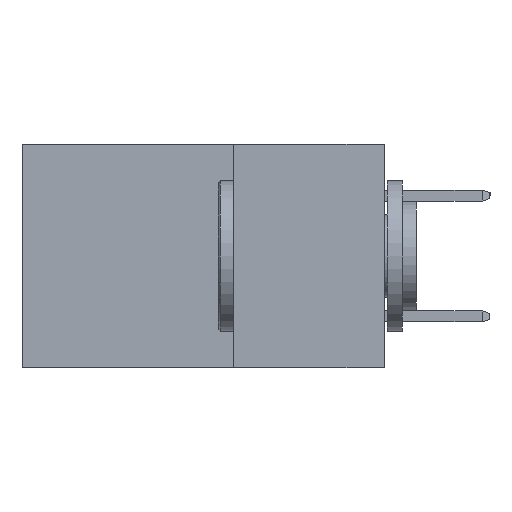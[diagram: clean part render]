
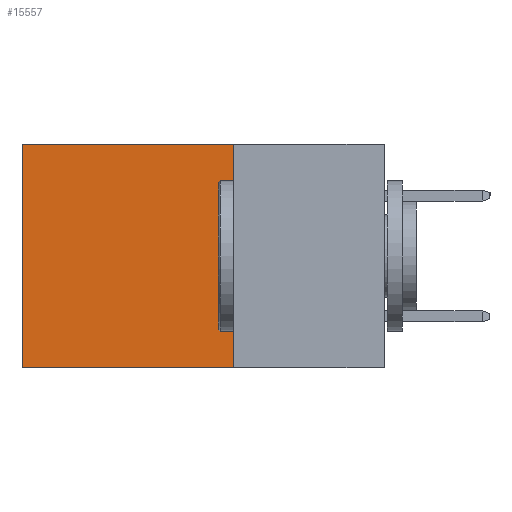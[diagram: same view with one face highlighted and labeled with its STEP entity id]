
A CAD part, left-side view. The second image highlights one B-rep face of the part: STEP entity #15557.
In plain terms, the highlighted planar face has unit normal (-1, 0, 0).
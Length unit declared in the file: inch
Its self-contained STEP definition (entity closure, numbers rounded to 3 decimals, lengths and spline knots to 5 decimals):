
#324 = VERTEX_POINT ( 'NONE', #13105 ) ;
#539 = DIRECTION ( 'NONE',  ( 1., 0., 0. ) ) ;
#744 = DIRECTION ( 'NONE',  ( 0., 0., -1. ) ) ;
#810 = EDGE_CURVE ( 'NONE', #5571, #15168, #15516, .T. ) ;
#1062 = CARTESIAN_POINT ( 'NONE',  ( 0.2615, 0.6, 0. ) ) ;
#1298 = VERTEX_POINT ( 'NONE', #1062 ) ;
#1554 = AXIS2_PLACEMENT_3D ( 'NONE', #6932, #539, #11868 ) ;
#1973 = EDGE_LOOP ( 'NONE', ( #11435, #13195, #6058, #9159 ) ) ;
#2013 = FACE_OUTER_BOUND ( 'NONE', #1973, .T. ) ;
#2723 = VECTOR ( 'NONE', #8713, 39.37008 ) ;
#3273 = VECTOR ( 'NONE', #15619, 39.37008 ) ;
#3799 = VECTOR ( 'NONE', #744, 39.37008 ) ;
#4315 = PLANE ( 'NONE',  #1554 ) ;
#5499 = EDGE_CURVE ( 'NONE', #15168, #324, #9925, .T. ) ;
#5571 = VERTEX_POINT ( 'NONE', #10310 ) ;
#6058 = ORIENTED_EDGE ( 'NONE', *, *, #810, .F. ) ;
#6932 = CARTESIAN_POINT ( 'NONE',  ( 0.2615, 0.25, -0.37 ) ) ;
#7161 = VECTOR ( 'NONE', #15175, 39.37008 ) ;
#8713 = DIRECTION ( 'NONE',  ( 0., 1., 0. ) ) ;
#9159 = ORIENTED_EDGE ( 'NONE', *, *, #10652, .T. ) ;
#9925 = LINE ( 'NONE', #14848, #2723 ) ;
#10310 = CARTESIAN_POINT ( 'NONE',  ( 0.2615, 0.25, 0. ) ) ;
#10652 = EDGE_CURVE ( 'NONE', #5571, #1298, #10810, .T. ) ;
#10810 = LINE ( 'NONE', #13281, #3273 ) ;
#11435 = ORIENTED_EDGE ( 'NONE', *, *, #13009, .T. ) ;
#11828 = CARTESIAN_POINT ( 'NONE',  ( 0.2615, 0.6, -0.37 ) ) ;
#11868 = DIRECTION ( 'NONE',  ( 0., 0., -1. ) ) ;
#13009 = EDGE_CURVE ( 'NONE', #1298, #324, #14633, .T. ) ;
#13105 = CARTESIAN_POINT ( 'NONE',  ( 0.2615, 0.6, -0.37 ) ) ;
#13195 = ORIENTED_EDGE ( 'NONE', *, *, #5499, .F. ) ;
#13281 = CARTESIAN_POINT ( 'NONE',  ( 0.2615, 0.25, 0. ) ) ;
#14633 = LINE ( 'NONE', #11828, #3799 ) ;
#14848 = CARTESIAN_POINT ( 'NONE',  ( 0.2615, 0.25, -0.37 ) ) ;
#15168 = VERTEX_POINT ( 'NONE', #15394 ) ;
#15175 = DIRECTION ( 'NONE',  ( 0., 0., -1. ) ) ;
#15265 = CARTESIAN_POINT ( 'NONE',  ( 0.2615, 0.25, -0.37 ) ) ;
#15394 = CARTESIAN_POINT ( 'NONE',  ( 0.2615, 0.25, -0.37 ) ) ;
#15516 = LINE ( 'NONE', #15265, #7161 ) ;
#15557 = ADVANCED_FACE ( 'NONE', ( #2013 ), #4315, .F. ) ;
#15619 = DIRECTION ( 'NONE',  ( 0., 1., 0. ) ) ;
